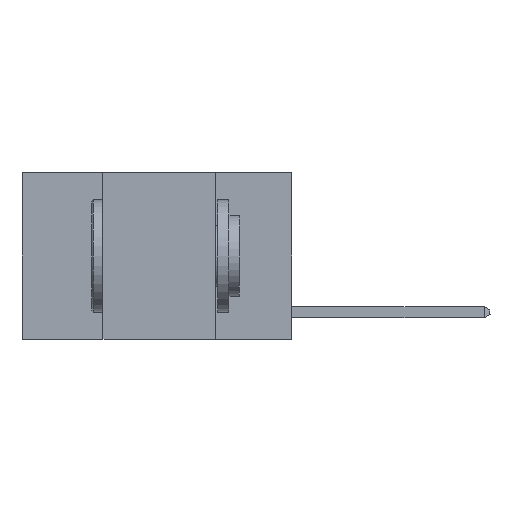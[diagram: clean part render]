
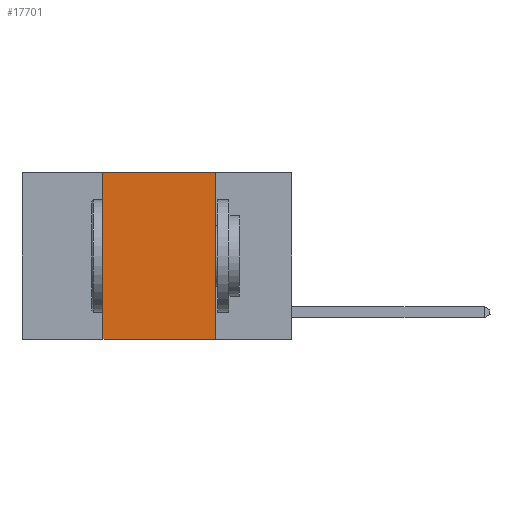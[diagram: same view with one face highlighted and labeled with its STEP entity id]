
A CAD part, left-side view. The second image highlights one B-rep face of the part: STEP entity #17701.
In plain terms, the highlighted planar face has unit normal (-1, 0, 0).
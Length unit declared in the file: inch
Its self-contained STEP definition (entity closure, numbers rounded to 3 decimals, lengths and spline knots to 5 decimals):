
#730 = CARTESIAN_POINT ( 'NONE',  ( 0., 0.6, 0. ) ) ;
#884 = EDGE_CURVE ( 'NONE', #11984, #9769, #20548, .T. ) ;
#952 = LINE ( 'NONE', #730, #21358 ) ;
#1429 = DIRECTION ( 'NONE',  ( 0., 0., -1. ) ) ;
#2181 = AXIS2_PLACEMENT_3D ( 'NONE', #19271, #15566, #1429 ) ;
#2903 = VERTEX_POINT ( 'NONE', #21796 ) ;
#3492 = FACE_OUTER_BOUND ( 'NONE', #14955, .T. ) ;
#4284 = DIRECTION ( 'NONE',  ( 0., 0., -1. ) ) ;
#5365 = EDGE_CURVE ( 'NONE', #11984, #2903, #12026, .T. ) ;
#6013 = CARTESIAN_POINT ( 'NONE',  ( 0., 0.17, -0.37 ) ) ;
#6273 = ORIENTED_EDGE ( 'NONE', *, *, #884, .T. ) ;
#7885 = DIRECTION ( 'NONE',  ( 0., -1., 0. ) ) ;
#8149 = ORIENTED_EDGE ( 'NONE', *, *, #16604, .F. ) ;
#9769 = VERTEX_POINT ( 'NONE', #6013 ) ;
#10058 = DIRECTION ( 'NONE',  ( 0., 0., 1. ) ) ;
#10219 = VECTOR ( 'NONE', #19998, 39.37008 ) ;
#11115 = CARTESIAN_POINT ( 'NONE',  ( 0., 0.17, 0. ) ) ;
#11716 = CARTESIAN_POINT ( 'NONE',  ( 0., 0.6, -0.37 ) ) ;
#11984 = VERTEX_POINT ( 'NONE', #16515 ) ;
#12026 = LINE ( 'NONE', #14005, #20437 ) ;
#12662 = ORIENTED_EDGE ( 'NONE', *, *, #5365, .F. ) ;
#13202 = LINE ( 'NONE', #11115, #19177 ) ;
#13543 = EDGE_CURVE ( 'NONE', #2903, #18003, #952, .T. ) ;
#14005 = CARTESIAN_POINT ( 'NONE',  ( 0., 0.42, 0. ) ) ;
#14955 = EDGE_LOOP ( 'NONE', ( #8149, #18180, #12662, #6273 ) ) ;
#15566 = DIRECTION ( 'NONE',  ( 1., 0., 0. ) ) ;
#16515 = CARTESIAN_POINT ( 'NONE',  ( 0., 0.42, -0.37 ) ) ;
#16604 = EDGE_CURVE ( 'NONE', #18003, #9769, #13202, .T. ) ;
#17701 = ADVANCED_FACE ( 'NONE', ( #3492 ), #22548, .F. ) ;
#18003 = VERTEX_POINT ( 'NONE', #20739 ) ;
#18180 = ORIENTED_EDGE ( 'NONE', *, *, #13543, .F. ) ;
#19177 = VECTOR ( 'NONE', #4284, 39.37008 ) ;
#19271 = CARTESIAN_POINT ( 'NONE',  ( 0., 0.6, 0. ) ) ;
#19998 = DIRECTION ( 'NONE',  ( 0., -1., 0. ) ) ;
#20437 = VECTOR ( 'NONE', #10058, 39.37008 ) ;
#20548 = LINE ( 'NONE', #11716, #10219 ) ;
#20739 = CARTESIAN_POINT ( 'NONE',  ( 0., 0.17, 0. ) ) ;
#21358 = VECTOR ( 'NONE', #7885, 39.37008 ) ;
#21796 = CARTESIAN_POINT ( 'NONE',  ( 0., 0.42, 0. ) ) ;
#22548 = PLANE ( 'NONE',  #2181 ) ;
